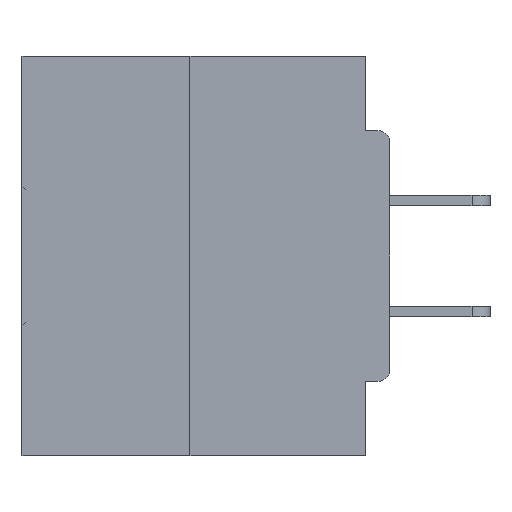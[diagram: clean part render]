
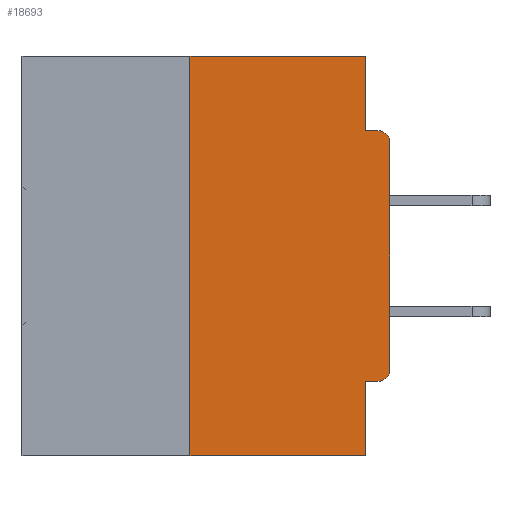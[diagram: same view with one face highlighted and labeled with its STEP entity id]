
A CAD part, left-side view. The second image highlights one B-rep face of the part: STEP entity #18693.
In plain terms, the highlighted planar face has unit normal (-1, 0, 0).
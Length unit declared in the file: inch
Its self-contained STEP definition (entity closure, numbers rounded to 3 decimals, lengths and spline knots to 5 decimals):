
#638 = EDGE_CURVE ( 'NONE', #30091, #34319, #9355, .T. ) ;
#928 = VECTOR ( 'NONE', #31858, 39.37008 ) ;
#3119 = EDGE_CURVE ( 'NONE', #33184, #6162, #9638, .T. ) ;
#4913 = VECTOR ( 'NONE', #40752, 39.37008 ) ;
#4984 = ORIENTED_EDGE ( 'NONE', *, *, #9423, .T. ) ;
#5057 = DIRECTION ( 'NONE',  ( 1., 0., 0. ) ) ;
#6012 = VERTEX_POINT ( 'NONE', #37599 ) ;
#6162 = VERTEX_POINT ( 'NONE', #34695 ) ;
#6483 = LINE ( 'NONE', #22601, #928 ) ;
#7324 = DIRECTION ( 'NONE',  ( 0., 0., -1. ) ) ;
#7830 = CARTESIAN_POINT ( 'NONE',  ( 0., 0.25, 0. ) ) ;
#8239 = DIRECTION ( 'NONE',  ( 0., 1., 0. ) ) ;
#8255 = VERTEX_POINT ( 'NONE', #8797 ) ;
#8797 = CARTESIAN_POINT ( 'NONE',  ( 0., 0., -0.3915 ) ) ;
#9355 = LINE ( 'NONE', #13585, #30410 ) ;
#9423 = EDGE_CURVE ( 'NONE', #20547, #6162, #15694, .T. ) ;
#9638 = LINE ( 'NONE', #24546, #24162 ) ;
#9953 = ORIENTED_EDGE ( 'NONE', *, *, #11995, .F. ) ;
#10074 = AXIS2_PLACEMENT_3D ( 'NONE', #26759, #20431, #33444 ) ;
#10089 = AXIS2_PLACEMENT_3D ( 'NONE', #21109, #5057, #40586 ) ;
#10755 = CARTESIAN_POINT ( 'NONE',  ( 0., 0., 0. ) ) ;
#10883 = DIRECTION ( 'NONE',  ( 0., 0., 1. ) ) ;
#11321 = PLANE ( 'NONE',  #10089 ) ;
#11861 = CARTESIAN_POINT ( 'NONE',  ( 0., 0.031, -0.0935 ) ) ;
#11995 = EDGE_CURVE ( 'NONE', #26612, #25610, #6483, .T. ) ;
#12270 = VECTOR ( 'NONE', #32507, 39.37008 ) ;
#12464 = CARTESIAN_POINT ( 'NONE',  ( 0., 0.015, -0.3915 ) ) ;
#12821 = EDGE_CURVE ( 'NONE', #6012, #34319, #25931, .T. ) ;
#13567 = CARTESIAN_POINT ( 'NONE',  ( 0., 0.031, 0. ) ) ;
#13585 = CARTESIAN_POINT ( 'NONE',  ( 0., 0.031, -0.5 ) ) ;
#14493 = ORIENTED_EDGE ( 'NONE', *, *, #638, .F. ) ;
#15496 = EDGE_LOOP ( 'NONE', ( #9953, #20543, #34583, #14493, #15704, #22862, #37029, #4984, #28490, #15898 ) ) ;
#15694 = CIRCLE ( 'NONE', #10074, 0.015 ) ;
#15704 = ORIENTED_EDGE ( 'NONE', *, *, #28779, .F. ) ;
#15898 = ORIENTED_EDGE ( 'NONE', *, *, #36981, .F. ) ;
#16343 = CARTESIAN_POINT ( 'NONE',  ( 0., 0.031, -0.5 ) ) ;
#16940 = CARTESIAN_POINT ( 'NONE',  ( 0., 0.25, 0. ) ) ;
#17208 = AXIS2_PLACEMENT_3D ( 'NONE', #12464, #34869, #22130 ) ;
#17463 = DIRECTION ( 'NONE',  ( 0., 0., 1. ) ) ;
#17986 = EDGE_CURVE ( 'NONE', #8255, #20547, #23063, .T. ) ;
#18693 = ADVANCED_FACE ( 'NONE', ( #39007 ), #11321, .F. ) ;
#19431 = VERTEX_POINT ( 'NONE', #28612 ) ;
#20431 = DIRECTION ( 'NONE',  ( -1., 0., 0. ) ) ;
#20543 = ORIENTED_EDGE ( 'NONE', *, *, #30215, .F. ) ;
#20547 = VERTEX_POINT ( 'NONE', #30427 ) ;
#21109 = CARTESIAN_POINT ( 'NONE',  ( 0., 0.46, 0. ) ) ;
#22130 = DIRECTION ( 'NONE',  ( 0., 0., -1. ) ) ;
#22601 = CARTESIAN_POINT ( 'NONE',  ( 0., 0.46, 0. ) ) ;
#22862 = ORIENTED_EDGE ( 'NONE', *, *, #27631, .T. ) ;
#23063 = LINE ( 'NONE', #10755, #26558 ) ;
#24162 = VECTOR ( 'NONE', #30703, 39.37008 ) ;
#24546 = CARTESIAN_POINT ( 'NONE',  ( 0., 0., -0.0935 ) ) ;
#25610 = VERTEX_POINT ( 'NONE', #13567 ) ;
#25931 = LINE ( 'NONE', #37788, #4913 ) ;
#26558 = VECTOR ( 'NONE', #17463, 39.37008 ) ;
#26612 = VERTEX_POINT ( 'NONE', #16940 ) ;
#26759 = CARTESIAN_POINT ( 'NONE',  ( 0., 0.015, -0.1085 ) ) ;
#27631 = EDGE_CURVE ( 'NONE', #19431, #8255, #35095, .T. ) ;
#27795 = LINE ( 'NONE', #32368, #12270 ) ;
#28391 = LINE ( 'NONE', #7830, #34858 ) ;
#28490 = ORIENTED_EDGE ( 'NONE', *, *, #3119, .F. ) ;
#28612 = CARTESIAN_POINT ( 'NONE',  ( 0., 0.015, -0.4065 ) ) ;
#28779 = EDGE_CURVE ( 'NONE', #19431, #30091, #31508, .T. ) ;
#30091 = VERTEX_POINT ( 'NONE', #32859 ) ;
#30215 = EDGE_CURVE ( 'NONE', #6012, #26612, #28391, .T. ) ;
#30410 = VECTOR ( 'NONE', #7324, 39.37008 ) ;
#30427 = CARTESIAN_POINT ( 'NONE',  ( 0., 0., -0.1085 ) ) ;
#30703 = DIRECTION ( 'NONE',  ( 0., -1., 0. ) ) ;
#31508 = LINE ( 'NONE', #33405, #39556 ) ;
#31858 = DIRECTION ( 'NONE',  ( 0., -1., 0. ) ) ;
#32368 = CARTESIAN_POINT ( 'NONE',  ( 0., 0.031, 0. ) ) ;
#32507 = DIRECTION ( 'NONE',  ( 0., 0., -1. ) ) ;
#32859 = CARTESIAN_POINT ( 'NONE',  ( 0., 0.031, -0.4065 ) ) ;
#33184 = VERTEX_POINT ( 'NONE', #11861 ) ;
#33405 = CARTESIAN_POINT ( 'NONE',  ( 0., 0., -0.4065 ) ) ;
#33444 = DIRECTION ( 'NONE',  ( 0., 0., -1. ) ) ;
#34319 = VERTEX_POINT ( 'NONE', #16343 ) ;
#34583 = ORIENTED_EDGE ( 'NONE', *, *, #12821, .T. ) ;
#34695 = CARTESIAN_POINT ( 'NONE',  ( 0., 0.015, -0.0935 ) ) ;
#34858 = VECTOR ( 'NONE', #10883, 39.37008 ) ;
#34869 = DIRECTION ( 'NONE',  ( -1., 0., 0. ) ) ;
#35095 = CIRCLE ( 'NONE', #17208, 0.015 ) ;
#36981 = EDGE_CURVE ( 'NONE', #25610, #33184, #27795, .T. ) ;
#37029 = ORIENTED_EDGE ( 'NONE', *, *, #17986, .T. ) ;
#37599 = CARTESIAN_POINT ( 'NONE',  ( 0., 0.25, -0.5 ) ) ;
#37788 = CARTESIAN_POINT ( 'NONE',  ( 0., 0.46, -0.5 ) ) ;
#39007 = FACE_OUTER_BOUND ( 'NONE', #15496, .T. ) ;
#39556 = VECTOR ( 'NONE', #8239, 39.37008 ) ;
#40586 = DIRECTION ( 'NONE',  ( 0., 0., -1. ) ) ;
#40752 = DIRECTION ( 'NONE',  ( 0., -1., 0. ) ) ;
